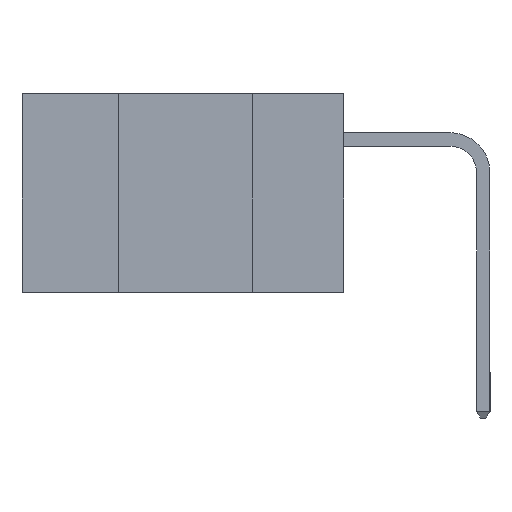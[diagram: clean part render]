
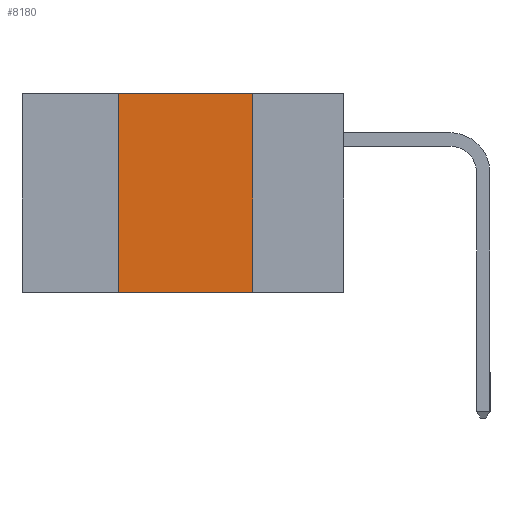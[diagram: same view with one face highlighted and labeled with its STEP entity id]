
A CAD part, left-side view. The second image highlights one B-rep face of the part: STEP entity #8180.
In plain terms, the highlighted planar face has unit normal (-1, 0, 0).
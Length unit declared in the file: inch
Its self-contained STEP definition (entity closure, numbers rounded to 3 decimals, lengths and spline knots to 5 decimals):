
#231 = LINE ( 'NONE', #17651, #7152 ) ;
#435 = CARTESIAN_POINT ( 'NONE',  ( 0., 0.6, 0. ) ) ;
#1915 = DIRECTION ( 'NONE',  ( 0., 0., 1. ) ) ;
#2211 = DIRECTION ( 'NONE',  ( 0., 0., -1. ) ) ;
#2411 = FACE_OUTER_BOUND ( 'NONE', #12675, .T. ) ;
#3204 = VECTOR ( 'NONE', #1915, 39.37008 ) ;
#3788 = PLANE ( 'NONE',  #15203 ) ;
#3905 = CARTESIAN_POINT ( 'NONE',  ( 0., 0.42, -0.37 ) ) ;
#3982 = LINE ( 'NONE', #13384, #16126 ) ;
#3986 = DIRECTION ( 'NONE',  ( 1., 0., 0. ) ) ;
#4631 = ORIENTED_EDGE ( 'NONE', *, *, #19960, .F. ) ;
#5353 = LINE ( 'NONE', #14657, #8534 ) ;
#7152 = VECTOR ( 'NONE', #18056, 39.37008 ) ;
#8180 = ADVANCED_FACE ( 'NONE', ( #2411 ), #3788, .F. ) ;
#8483 = DIRECTION ( 'NONE',  ( 0., 0., -1. ) ) ;
#8534 = VECTOR ( 'NONE', #8601, 39.37008 ) ;
#8601 = DIRECTION ( 'NONE',  ( 0., -1., 0. ) ) ;
#10808 = EDGE_CURVE ( 'NONE', #14520, #12994, #231, .T. ) ;
#10993 = EDGE_CURVE ( 'NONE', #14717, #12994, #3982, .T. ) ;
#11149 = ORIENTED_EDGE ( 'NONE', *, *, #10993, .F. ) ;
#12675 = EDGE_LOOP ( 'NONE', ( #11149, #19766, #4631, #15932 ) ) ;
#12994 = VERTEX_POINT ( 'NONE', #18858 ) ;
#13384 = CARTESIAN_POINT ( 'NONE',  ( 0., 0.17, -0.37 ) ) ;
#14520 = VERTEX_POINT ( 'NONE', #15178 ) ;
#14632 = CARTESIAN_POINT ( 'NONE',  ( 0., 0.17, 0. ) ) ;
#14657 = CARTESIAN_POINT ( 'NONE',  ( 0., 0.6, 0. ) ) ;
#14717 = VERTEX_POINT ( 'NONE', #14632 ) ;
#15178 = CARTESIAN_POINT ( 'NONE',  ( 0., 0.42, -0.37 ) ) ;
#15203 = AXIS2_PLACEMENT_3D ( 'NONE', #435, #3986, #8483 ) ;
#15932 = ORIENTED_EDGE ( 'NONE', *, *, #10808, .T. ) ;
#16126 = VECTOR ( 'NONE', #2211, 39.37008 ) ;
#17651 = CARTESIAN_POINT ( 'NONE',  ( 0., 0.6, -0.37 ) ) ;
#17878 = CARTESIAN_POINT ( 'NONE',  ( 0., 0.42, 0. ) ) ;
#18056 = DIRECTION ( 'NONE',  ( 0., -1., 0. ) ) ;
#18161 = VERTEX_POINT ( 'NONE', #17878 ) ;
#18184 = LINE ( 'NONE', #3905, #3204 ) ;
#18858 = CARTESIAN_POINT ( 'NONE',  ( 0., 0.17, -0.37 ) ) ;
#19766 = ORIENTED_EDGE ( 'NONE', *, *, #19992, .F. ) ;
#19960 = EDGE_CURVE ( 'NONE', #14520, #18161, #18184, .T. ) ;
#19992 = EDGE_CURVE ( 'NONE', #18161, #14717, #5353, .T. ) ;
